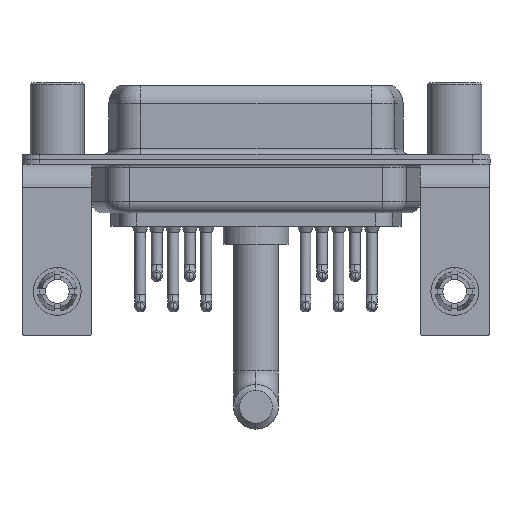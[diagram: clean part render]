
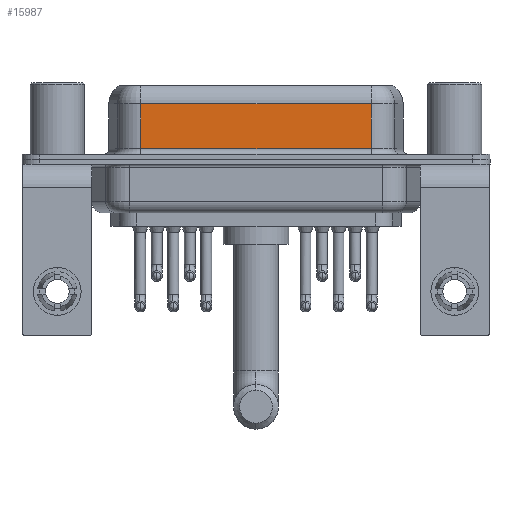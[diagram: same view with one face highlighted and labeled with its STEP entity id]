
A CAD part, front view. The second image highlights one B-rep face of the part: STEP entity #15987.
In plain terms, the highlighted planar face has unit normal (0, -1, 0).
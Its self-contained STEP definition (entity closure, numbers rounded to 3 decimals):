
#357 = VERTEX_POINT ( 'NONE', #12245 ) ;
#413 = CARTESIAN_POINT ( 'NONE',  ( 7.013, -3.95, 4.65 ) ) ;
#639 = CARTESIAN_POINT ( 'NONE',  ( 26.287, -3.95, 4.65 ) ) ;
#1168 = DIRECTION ( 'NONE',  ( -1., 0., 0. ) ) ;
#1469 = DIRECTION ( 'NONE',  ( 0., 0., 1. ) ) ;
#1670 = EDGE_LOOP ( 'NONE', ( #16324, #21954, #7121, #8036 ) ) ;
#3048 = VECTOR ( 'NONE', #9526, 1000. ) ;
#3294 = CARTESIAN_POINT ( 'NONE',  ( 7.013, -3.95, 0.9 ) ) ;
#3751 = DIRECTION ( 'NONE',  ( 0., 0., -1. ) ) ;
#3865 = CARTESIAN_POINT ( 'NONE',  ( 26.287, -3.95, 0.9 ) ) ;
#3868 = CARTESIAN_POINT ( 'NONE',  ( 7.013, -3.95, 6.4 ) ) ;
#4718 = VECTOR ( 'NONE', #3751, 1000. ) ;
#5157 = PLANE ( 'NONE',  #5242 ) ;
#5242 = AXIS2_PLACEMENT_3D ( 'NONE', #14931, #17072, #1469 ) ;
#7121 = ORIENTED_EDGE ( 'NONE', *, *, #11236, .T. ) ;
#7441 = VERTEX_POINT ( 'NONE', #639 ) ;
#8036 = ORIENTED_EDGE ( 'NONE', *, *, #17446, .T. ) ;
#8312 = VERTEX_POINT ( 'NONE', #3294 ) ;
#8662 = VERTEX_POINT ( 'NONE', #413 ) ;
#9466 = EDGE_CURVE ( 'NONE', #7441, #8662, #14741, .T. ) ;
#9526 = DIRECTION ( 'NONE',  ( 0., 0., -1. ) ) ;
#11236 = EDGE_CURVE ( 'NONE', #8662, #8312, #14194, .T. ) ;
#11892 = FACE_OUTER_BOUND ( 'NONE', #1670, .T. ) ;
#12245 = CARTESIAN_POINT ( 'NONE',  ( 26.287, -3.95, 0.9 ) ) ;
#12390 = LINE ( 'NONE', #3865, #20736 ) ;
#12787 = CARTESIAN_POINT ( 'NONE',  ( 26.287, -3.95, 6.4 ) ) ;
#14194 = LINE ( 'NONE', #3868, #4718 ) ;
#14741 = LINE ( 'NONE', #18248, #17627 ) ;
#14931 = CARTESIAN_POINT ( 'NONE',  ( 26.287, -3.95, 6.4 ) ) ;
#15987 = ADVANCED_FACE ( 'NONE', ( #11892 ), #5157, .F. ) ;
#16324 = ORIENTED_EDGE ( 'NONE', *, *, #16447, .F. ) ;
#16447 = EDGE_CURVE ( 'NONE', #7441, #357, #21674, .T. ) ;
#17072 = DIRECTION ( 'NONE',  ( 0., 1., 0. ) ) ;
#17446 = EDGE_CURVE ( 'NONE', #8312, #357, #12390, .T. ) ;
#17627 = VECTOR ( 'NONE', #1168, 1000. ) ;
#17914 = DIRECTION ( 'NONE',  ( 1., 0., 0. ) ) ;
#18248 = CARTESIAN_POINT ( 'NONE',  ( 26.287, -3.95, 4.65 ) ) ;
#20736 = VECTOR ( 'NONE', #17914, 1000. ) ;
#21674 = LINE ( 'NONE', #12787, #3048 ) ;
#21954 = ORIENTED_EDGE ( 'NONE', *, *, #9466, .T. ) ;
